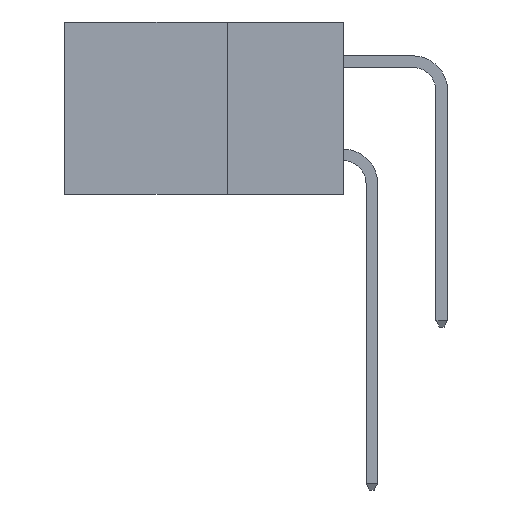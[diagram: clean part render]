
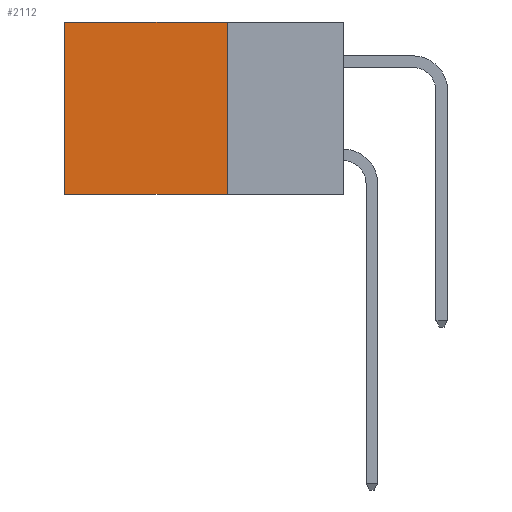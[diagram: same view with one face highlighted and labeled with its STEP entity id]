
A CAD part, left-side view. The second image highlights one B-rep face of the part: STEP entity #2112.
In plain terms, the highlighted planar face has unit normal (-1, 0, 0).
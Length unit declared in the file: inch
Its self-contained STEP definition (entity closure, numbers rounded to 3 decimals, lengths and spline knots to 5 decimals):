
#878 = VECTOR ( 'NONE', #14597, 39.37008 ) ;
#1942 = EDGE_CURVE ( 'NONE', #13095, #5582, #2709, .T. ) ;
#2112 = ADVANCED_FACE ( 'NONE', ( #6517 ), #14158, .F. ) ;
#2709 = LINE ( 'NONE', #11369, #11663 ) ;
#2871 = EDGE_LOOP ( 'NONE', ( #12707, #11812, #9265, #14204 ) ) ;
#3032 = VERTEX_POINT ( 'NONE', #10400 ) ;
#5029 = DIRECTION ( 'NONE',  ( 0., 1., 0. ) ) ;
#5126 = CARTESIAN_POINT ( 'NONE',  ( 0.2615, 0.25, -0.37 ) ) ;
#5582 = VERTEX_POINT ( 'NONE', #8808 ) ;
#6517 = FACE_OUTER_BOUND ( 'NONE', #2871, .T. ) ;
#7191 = EDGE_CURVE ( 'NONE', #5582, #3032, #11083, .T. ) ;
#7485 = LINE ( 'NONE', #13468, #878 ) ;
#8249 = AXIS2_PLACEMENT_3D ( 'NONE', #14719, #14535, #14516 ) ;
#8620 = VERTEX_POINT ( 'NONE', #14843 ) ;
#8808 = CARTESIAN_POINT ( 'NONE',  ( 0.2615, 0.25, -0.37 ) ) ;
#8836 = EDGE_CURVE ( 'NONE', #13095, #8620, #14161, .T. ) ;
#9265 = ORIENTED_EDGE ( 'NONE', *, *, #1942, .F. ) ;
#9453 = CARTESIAN_POINT ( 'NONE',  ( 0.2615, 0.25, 0. ) ) ;
#10400 = CARTESIAN_POINT ( 'NONE',  ( 0.2615, 0.6, -0.37 ) ) ;
#10688 = DIRECTION ( 'NONE',  ( 0., 1., 0. ) ) ;
#10880 = CARTESIAN_POINT ( 'NONE',  ( 0.2615, 0.25, 0. ) ) ;
#11083 = LINE ( 'NONE', #5126, #11446 ) ;
#11369 = CARTESIAN_POINT ( 'NONE',  ( 0.2615, 0.25, -0.37 ) ) ;
#11446 = VECTOR ( 'NONE', #5029, 39.37008 ) ;
#11663 = VECTOR ( 'NONE', #13585, 39.37008 ) ;
#11812 = ORIENTED_EDGE ( 'NONE', *, *, #7191, .F. ) ;
#12707 = ORIENTED_EDGE ( 'NONE', *, *, #13989, .T. ) ;
#13095 = VERTEX_POINT ( 'NONE', #9453 ) ;
#13468 = CARTESIAN_POINT ( 'NONE',  ( 0.2615, 0.6, -0.37 ) ) ;
#13585 = DIRECTION ( 'NONE',  ( 0., 0., -1. ) ) ;
#13809 = VECTOR ( 'NONE', #10688, 39.37008 ) ;
#13989 = EDGE_CURVE ( 'NONE', #8620, #3032, #7485, .T. ) ;
#14158 = PLANE ( 'NONE',  #8249 ) ;
#14161 = LINE ( 'NONE', #10880, #13809 ) ;
#14204 = ORIENTED_EDGE ( 'NONE', *, *, #8836, .T. ) ;
#14516 = DIRECTION ( 'NONE',  ( 0., 0., -1. ) ) ;
#14535 = DIRECTION ( 'NONE',  ( 1., 0., 0. ) ) ;
#14597 = DIRECTION ( 'NONE',  ( 0., 0., -1. ) ) ;
#14719 = CARTESIAN_POINT ( 'NONE',  ( 0.2615, 0.25, -0.37 ) ) ;
#14843 = CARTESIAN_POINT ( 'NONE',  ( 0.2615, 0.6, 0. ) ) ;
